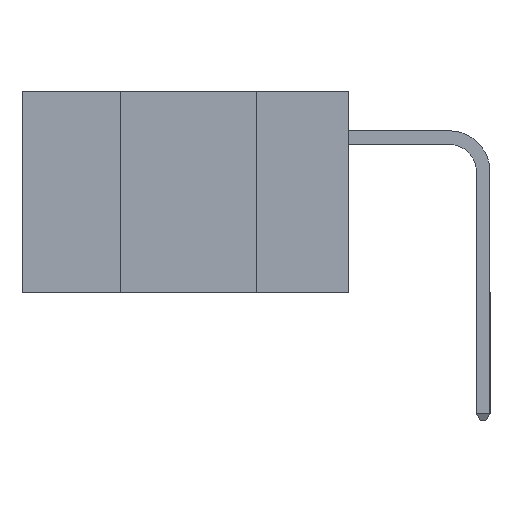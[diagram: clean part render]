
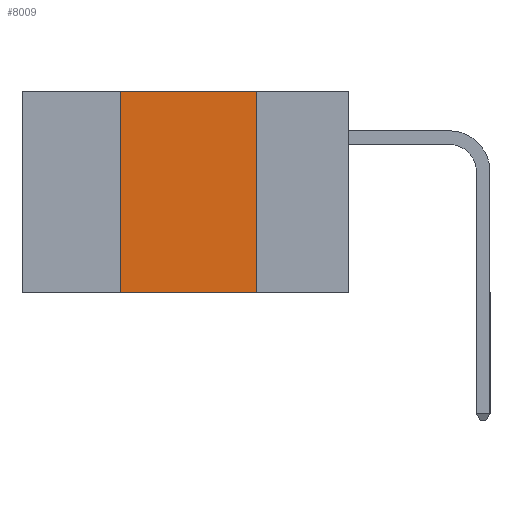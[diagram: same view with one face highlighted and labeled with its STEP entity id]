
A CAD part, left-side view. The second image highlights one B-rep face of the part: STEP entity #8009.
In plain terms, the highlighted planar face has unit normal (-1, 0, 0).
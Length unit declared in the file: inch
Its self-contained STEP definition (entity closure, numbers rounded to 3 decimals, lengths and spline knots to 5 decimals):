
#12 = VERTEX_POINT ( 'NONE', #6548 ) ;
#2093 = LINE ( 'NONE', #9630, #10395 ) ;
#2485 = EDGE_CURVE ( 'NONE', #12, #10430, #2093, .T. ) ;
#3332 = EDGE_CURVE ( 'NONE', #10430, #7910, #8928, .T. ) ;
#3584 = LINE ( 'NONE', #6881, #9640 ) ;
#4179 = ORIENTED_EDGE ( 'NONE', *, *, #5462, .T. ) ;
#4272 = EDGE_LOOP ( 'NONE', ( #6739, #7937, #7281, #4179 ) ) ;
#4340 = PLANE ( 'NONE',  #6618 ) ;
#5182 = CARTESIAN_POINT ( 'NONE',  ( 0., 0.6, 0. ) ) ;
#5264 = EDGE_CURVE ( 'NONE', #9888, #12, #9019, .T. ) ;
#5384 = FACE_OUTER_BOUND ( 'NONE', #4272, .T. ) ;
#5462 = EDGE_CURVE ( 'NONE', #9888, #7910, #3584, .T. ) ;
#5600 = DIRECTION ( 'NONE',  ( 0., 0., -1. ) ) ;
#5698 = CARTESIAN_POINT ( 'NONE',  ( 0., 0.17, 0. ) ) ;
#5952 = DIRECTION ( 'NONE',  ( 0., 0., -1. ) ) ;
#6364 = CARTESIAN_POINT ( 'NONE',  ( 0., 0.17, 0. ) ) ;
#6548 = CARTESIAN_POINT ( 'NONE',  ( 0., 0.42, 0. ) ) ;
#6618 = AXIS2_PLACEMENT_3D ( 'NONE', #5182, #10557, #5952 ) ;
#6739 = ORIENTED_EDGE ( 'NONE', *, *, #3332, .F. ) ;
#6881 = CARTESIAN_POINT ( 'NONE',  ( 0., 0.6, -0.37 ) ) ;
#6891 = DIRECTION ( 'NONE',  ( 0., -1., 0. ) ) ;
#6986 = VECTOR ( 'NONE', #7596, 39.37008 ) ;
#7281 = ORIENTED_EDGE ( 'NONE', *, *, #5264, .F. ) ;
#7596 = DIRECTION ( 'NONE',  ( 0., 0., 1. ) ) ;
#7620 = CARTESIAN_POINT ( 'NONE',  ( 0., 0.42, 0. ) ) ;
#7801 = DIRECTION ( 'NONE',  ( 0., -1., 0. ) ) ;
#7910 = VERTEX_POINT ( 'NONE', #10004 ) ;
#7937 = ORIENTED_EDGE ( 'NONE', *, *, #2485, .F. ) ;
#8009 = ADVANCED_FACE ( 'NONE', ( #5384 ), #4340, .F. ) ;
#8928 = LINE ( 'NONE', #5698, #10725 ) ;
#9019 = LINE ( 'NONE', #7620, #6986 ) ;
#9240 = CARTESIAN_POINT ( 'NONE',  ( 0., 0.42, -0.37 ) ) ;
#9630 = CARTESIAN_POINT ( 'NONE',  ( 0., 0.6, 0. ) ) ;
#9640 = VECTOR ( 'NONE', #6891, 39.37008 ) ;
#9888 = VERTEX_POINT ( 'NONE', #9240 ) ;
#10004 = CARTESIAN_POINT ( 'NONE',  ( 0., 0.17, -0.37 ) ) ;
#10395 = VECTOR ( 'NONE', #7801, 39.37008 ) ;
#10430 = VERTEX_POINT ( 'NONE', #6364 ) ;
#10557 = DIRECTION ( 'NONE',  ( 1., 0., 0. ) ) ;
#10725 = VECTOR ( 'NONE', #5600, 39.37008 ) ;
